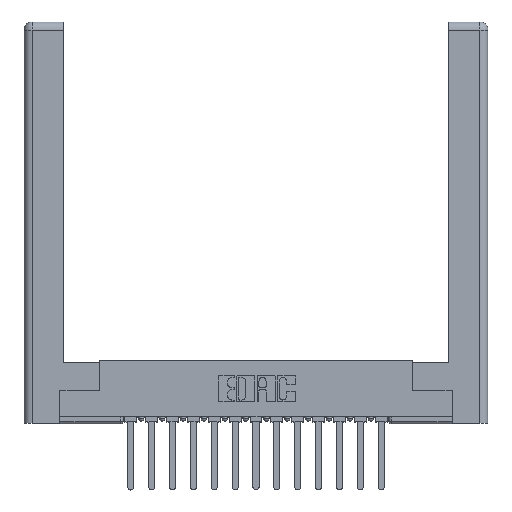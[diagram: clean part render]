
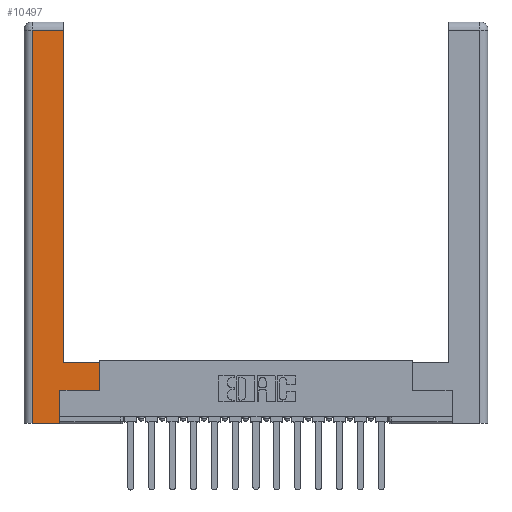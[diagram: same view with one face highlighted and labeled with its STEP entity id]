
A CAD part, top view. The second image highlights one B-rep face of the part: STEP entity #10497.
In plain terms, the highlighted planar face has unit normal (0, 0, 1).
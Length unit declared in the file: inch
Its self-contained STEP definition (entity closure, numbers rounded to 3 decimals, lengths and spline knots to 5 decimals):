
#4 = CARTESIAN_POINT ( 'NONE',  ( 0.265, 0., 0. ) ) ;
#191 = LINE ( 'NONE', #4906, #413 ) ;
#413 = VECTOR ( 'NONE', #7658, 39.37008 ) ;
#1050 = EDGE_LOOP ( 'NONE', ( #13066, #9751, #6574, #15440, #9548, #6057, #1722, #7340 ) ) ;
#1170 = CARTESIAN_POINT ( 'NONE',  ( 0., 0., 0. ) ) ;
#1404 = LINE ( 'NONE', #1411, #12939 ) ;
#1408 = CARTESIAN_POINT ( 'NONE',  ( 0.565, 0.245, 0. ) ) ;
#1411 = CARTESIAN_POINT ( 'NONE',  ( 0.265, 0.245, 0. ) ) ;
#1722 = ORIENTED_EDGE ( 'NONE', *, *, #8330, .T. ) ;
#2062 = EDGE_CURVE ( 'NONE', #9552, #11945, #191, .T. ) ;
#2090 = DIRECTION ( 'NONE',  ( -1., 0., 0. ) ) ;
#2387 = DIRECTION ( 'NONE',  ( 0., 1., 0. ) ) ;
#3059 = VERTEX_POINT ( 'NONE', #4469 ) ;
#3533 = CARTESIAN_POINT ( 'NONE',  ( 0.295, 0.45, 0. ) ) ;
#3566 = LINE ( 'NONE', #10239, #12249 ) ;
#4469 = CARTESIAN_POINT ( 'NONE',  ( 0.265, 0., 0. ) ) ;
#4906 = CARTESIAN_POINT ( 'NONE',  ( 0.565, 0.245, 0. ) ) ;
#4912 = EDGE_CURVE ( 'NONE', #5738, #16242, #15997, .T. ) ;
#4933 = EDGE_CURVE ( 'NONE', #12511, #5738, #3566, .T. ) ;
#5189 = LINE ( 'NONE', #3533, #11262 ) ;
#5738 = VERTEX_POINT ( 'NONE', #12761 ) ;
#6057 = ORIENTED_EDGE ( 'NONE', *, *, #2062, .T. ) ;
#6156 = VECTOR ( 'NONE', #16087, 39.37008 ) ;
#6262 = CARTESIAN_POINT ( 'NONE',  ( 0.0615, 0., 0. ) ) ;
#6574 = ORIENTED_EDGE ( 'NONE', *, *, #9173, .T. ) ;
#7340 = ORIENTED_EDGE ( 'NONE', *, *, #18004, .T. ) ;
#7658 = DIRECTION ( 'NONE',  ( 1., 0., 0. ) ) ;
#8246 = FACE_OUTER_BOUND ( 'NONE', #1050, .T. ) ;
#8330 = EDGE_CURVE ( 'NONE', #11945, #15648, #9644, .T. ) ;
#9173 = EDGE_CURVE ( 'NONE', #16242, #11594, #14678, .T. ) ;
#9548 = ORIENTED_EDGE ( 'NONE', *, *, #13732, .T. ) ;
#9552 = VERTEX_POINT ( 'NONE', #14175 ) ;
#9644 = LINE ( 'NONE', #9667, #13609 ) ;
#9667 = CARTESIAN_POINT ( 'NONE',  ( 0.565, 0.45, 0. ) ) ;
#9751 = ORIENTED_EDGE ( 'NONE', *, *, #4912, .T. ) ;
#10239 = CARTESIAN_POINT ( 'NONE',  ( 0.295, 3., 0. ) ) ;
#10497 = ADVANCED_FACE ( 'NONE', ( #8246 ), #10818, .F. ) ;
#10700 = CARTESIAN_POINT ( 'NONE',  ( 0.0615, 0., 0. ) ) ;
#10818 = PLANE ( 'NONE',  #14672 ) ;
#10885 = DIRECTION ( 'NONE',  ( 0., 0., -1. ) ) ;
#10896 = VECTOR ( 'NONE', #18058, 39.37008 ) ;
#11262 = VECTOR ( 'NONE', #2090, 39.37008 ) ;
#11594 = VERTEX_POINT ( 'NONE', #10700 ) ;
#11945 = VERTEX_POINT ( 'NONE', #1408 ) ;
#12249 = VECTOR ( 'NONE', #2387, 39.37008 ) ;
#12293 = DIRECTION ( 'NONE',  ( -1., 0., 0. ) ) ;
#12511 = VERTEX_POINT ( 'NONE', #13798 ) ;
#12551 = DIRECTION ( 'NONE',  ( 0., 1., 0. ) ) ;
#12761 = CARTESIAN_POINT ( 'NONE',  ( 0.295, 2.94, 0. ) ) ;
#12939 = VECTOR ( 'NONE', #14126, 39.37008 ) ;
#13066 = ORIENTED_EDGE ( 'NONE', *, *, #4933, .T. ) ;
#13235 = CARTESIAN_POINT ( 'NONE',  ( 0.0615, 2.94, 0. ) ) ;
#13609 = VECTOR ( 'NONE', #12551, 39.37008 ) ;
#13732 = EDGE_CURVE ( 'NONE', #3059, #9552, #1404, .T. ) ;
#13759 = LINE ( 'NONE', #4, #10896 ) ;
#13798 = CARTESIAN_POINT ( 'NONE',  ( 0.295, 0.45, 0. ) ) ;
#14126 = DIRECTION ( 'NONE',  ( 0., 1., 0. ) ) ;
#14175 = CARTESIAN_POINT ( 'NONE',  ( 0.265, 0.245, 0. ) ) ;
#14538 = CARTESIAN_POINT ( 'NONE',  ( 0.565, 0.45, 0. ) ) ;
#14672 = AXIS2_PLACEMENT_3D ( 'NONE', #1170, #10885, #12293 ) ;
#14678 = LINE ( 'NONE', #6262, #6156 ) ;
#15440 = ORIENTED_EDGE ( 'NONE', *, *, #16049, .T. ) ;
#15648 = VERTEX_POINT ( 'NONE', #14538 ) ;
#15807 = DIRECTION ( 'NONE',  ( -1., 0., 0. ) ) ;
#15997 = LINE ( 'NONE', #13235, #16867 ) ;
#16049 = EDGE_CURVE ( 'NONE', #11594, #3059, #13759, .T. ) ;
#16087 = DIRECTION ( 'NONE',  ( 0., -1., 0. ) ) ;
#16242 = VERTEX_POINT ( 'NONE', #17159 ) ;
#16867 = VECTOR ( 'NONE', #15807, 39.37008 ) ;
#17159 = CARTESIAN_POINT ( 'NONE',  ( 0.0615, 2.94, 0. ) ) ;
#18004 = EDGE_CURVE ( 'NONE', #15648, #12511, #5189, .T. ) ;
#18058 = DIRECTION ( 'NONE',  ( 1., 0., 0. ) ) ;
